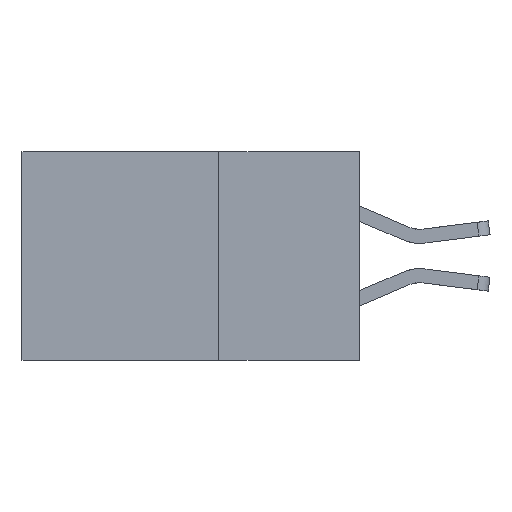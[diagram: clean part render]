
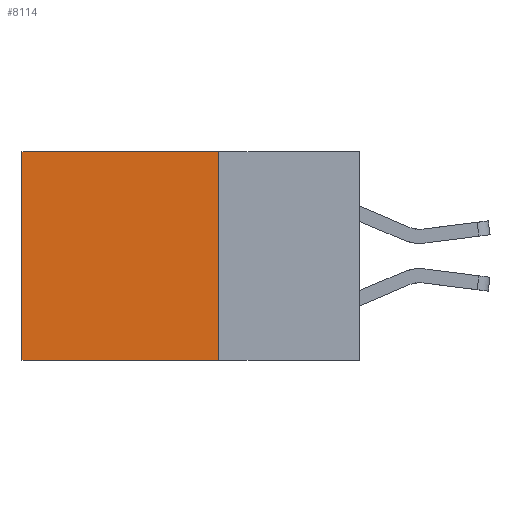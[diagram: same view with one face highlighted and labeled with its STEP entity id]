
A CAD part, left-side view. The second image highlights one B-rep face of the part: STEP entity #8114.
In plain terms, the highlighted planar face has unit normal (-1, 0, 0).
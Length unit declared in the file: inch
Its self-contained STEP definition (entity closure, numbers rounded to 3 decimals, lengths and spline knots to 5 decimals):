
#43 = FACE_OUTER_BOUND ( 'NONE', #7782, .T. ) ;
#179 = PLANE ( 'NONE',  #4243 ) ;
#431 = EDGE_CURVE ( 'NONE', #1617, #5325, #8983, .T. ) ;
#671 = CARTESIAN_POINT ( 'NONE',  ( 0.2875, 0.6, 0. ) ) ;
#898 = CARTESIAN_POINT ( 'NONE',  ( 0.2875, 0.25, 0. ) ) ;
#1143 = CARTESIAN_POINT ( 'NONE',  ( 0.2875, 0.25, -0.37 ) ) ;
#1211 = DIRECTION ( 'NONE',  ( 0., 1., 0. ) ) ;
#1617 = VERTEX_POINT ( 'NONE', #6899 ) ;
#1790 = DIRECTION ( 'NONE',  ( 0., 1., 0. ) ) ;
#1843 = CARTESIAN_POINT ( 'NONE',  ( 0.2875, 0.6, 0. ) ) ;
#2134 = VERTEX_POINT ( 'NONE', #8823 ) ;
#2917 = VECTOR ( 'NONE', #6205, 39.37008 ) ;
#3145 = VECTOR ( 'NONE', #1211, 39.37008 ) ;
#3363 = DIRECTION ( 'NONE',  ( 0., 0., -1. ) ) ;
#3595 = LINE ( 'NONE', #1843, #9455 ) ;
#3954 = DIRECTION ( 'NONE',  ( 1., 0., 0. ) ) ;
#3983 = VECTOR ( 'NONE', #1790, 39.37008 ) ;
#4052 = DIRECTION ( 'NONE',  ( 0., 0., -1. ) ) ;
#4243 = AXIS2_PLACEMENT_3D ( 'NONE', #5501, #3954, #4052 ) ;
#4460 = LINE ( 'NONE', #1143, #3145 ) ;
#5325 = VERTEX_POINT ( 'NONE', #671 ) ;
#5501 = CARTESIAN_POINT ( 'NONE',  ( 0.2875, 0.25, 0. ) ) ;
#5751 = ORIENTED_EDGE ( 'NONE', *, *, #431, .T. ) ;
#6153 = ORIENTED_EDGE ( 'NONE', *, *, #8404, .F. ) ;
#6205 = DIRECTION ( 'NONE',  ( 0., 0., -1. ) ) ;
#6899 = CARTESIAN_POINT ( 'NONE',  ( 0.2875, 0.25, 0. ) ) ;
#7343 = CARTESIAN_POINT ( 'NONE',  ( 0.2875, 0.25, -0.37 ) ) ;
#7782 = EDGE_LOOP ( 'NONE', ( #9611, #8056, #6153, #5751 ) ) ;
#8056 = ORIENTED_EDGE ( 'NONE', *, *, #8467, .F. ) ;
#8114 = ADVANCED_FACE ( 'NONE', ( #43 ), #179, .F. ) ;
#8404 = EDGE_CURVE ( 'NONE', #1617, #9713, #9239, .T. ) ;
#8467 = EDGE_CURVE ( 'NONE', #9713, #2134, #4460, .T. ) ;
#8823 = CARTESIAN_POINT ( 'NONE',  ( 0.2875, 0.6, -0.37 ) ) ;
#8983 = LINE ( 'NONE', #9449, #3983 ) ;
#9239 = LINE ( 'NONE', #898, #2917 ) ;
#9449 = CARTESIAN_POINT ( 'NONE',  ( 0.2875, 0.25, 0. ) ) ;
#9455 = VECTOR ( 'NONE', #3363, 39.37008 ) ;
#9611 = ORIENTED_EDGE ( 'NONE', *, *, #9613, .T. ) ;
#9613 = EDGE_CURVE ( 'NONE', #5325, #2134, #3595, .T. ) ;
#9713 = VERTEX_POINT ( 'NONE', #7343 ) ;
